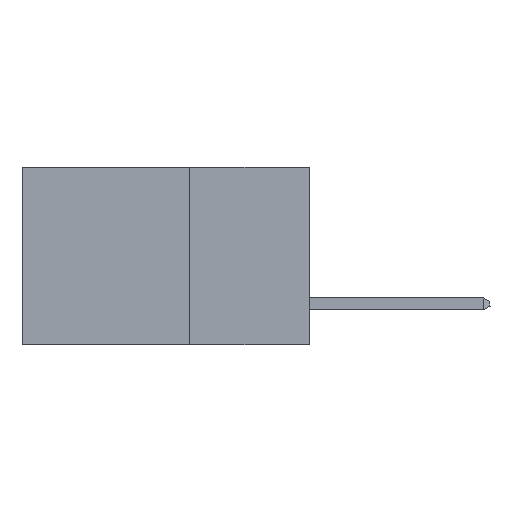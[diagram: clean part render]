
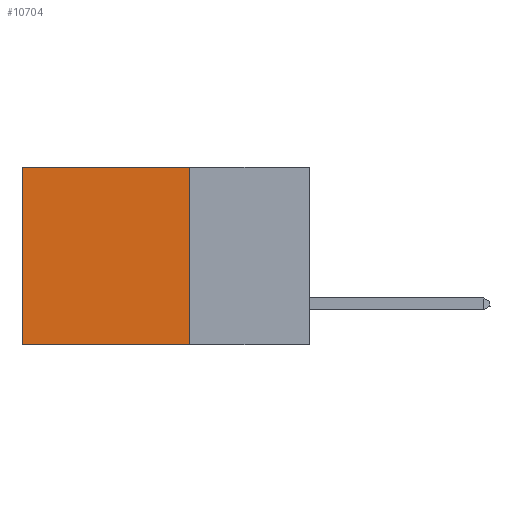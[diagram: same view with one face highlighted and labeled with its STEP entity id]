
A CAD part, left-side view. The second image highlights one B-rep face of the part: STEP entity #10704.
In plain terms, the highlighted planar face has unit normal (-1, 0, 0).
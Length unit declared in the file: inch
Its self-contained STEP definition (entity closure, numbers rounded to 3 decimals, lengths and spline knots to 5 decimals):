
#724 = LINE ( 'NONE', #19006, #25003 ) ;
#841 = CARTESIAN_POINT ( 'NONE',  ( 0.2875, 0.6, 0. ) ) ;
#2384 = CARTESIAN_POINT ( 'NONE',  ( 0.2875, 0.25, 0. ) ) ;
#4241 = ORIENTED_EDGE ( 'NONE', *, *, #12187, .T. ) ;
#4964 = VERTEX_POINT ( 'NONE', #38207 ) ;
#5717 = DIRECTION ( 'NONE',  ( 0., 0., -1. ) ) ;
#5896 = CARTESIAN_POINT ( 'NONE',  ( 0.2875, 0.25, -0.37 ) ) ;
#7204 = DIRECTION ( 'NONE',  ( 0., 1., 0. ) ) ;
#9213 = VERTEX_POINT ( 'NONE', #10234 ) ;
#10234 = CARTESIAN_POINT ( 'NONE',  ( 0.2875, 0.25, -0.37 ) ) ;
#10535 = VECTOR ( 'NONE', #20836, 39.37008 ) ;
#10704 = ADVANCED_FACE ( 'NONE', ( #17303 ), #29301, .F. ) ;
#11171 = CARTESIAN_POINT ( 'NONE',  ( 0.2875, 0.25, 0. ) ) ;
#11302 = VECTOR ( 'NONE', #21482, 39.37008 ) ;
#12187 = EDGE_CURVE ( 'NONE', #28673, #31275, #12631, .T. ) ;
#12631 = LINE ( 'NONE', #841, #11302 ) ;
#12704 = LINE ( 'NONE', #5896, #10535 ) ;
#15066 = VECTOR ( 'NONE', #22585, 39.37008 ) ;
#15431 = ORIENTED_EDGE ( 'NONE', *, *, #24665, .T. ) ;
#17303 = FACE_OUTER_BOUND ( 'NONE', #21551, .T. ) ;
#19006 = CARTESIAN_POINT ( 'NONE',  ( 0.2875, 0.25, 0. ) ) ;
#19145 = CARTESIAN_POINT ( 'NONE',  ( 0.2875, 0.6, 0. ) ) ;
#19817 = LINE ( 'NONE', #11171, #15066 ) ;
#20836 = DIRECTION ( 'NONE',  ( 0., 1., 0. ) ) ;
#21482 = DIRECTION ( 'NONE',  ( 0., 0., -1. ) ) ;
#21551 = EDGE_LOOP ( 'NONE', ( #4241, #22444, #23532, #15431 ) ) ;
#22118 = CARTESIAN_POINT ( 'NONE',  ( 0.2875, 0.6, -0.37 ) ) ;
#22444 = ORIENTED_EDGE ( 'NONE', *, *, #22811, .F. ) ;
#22585 = DIRECTION ( 'NONE',  ( 0., 0., -1. ) ) ;
#22811 = EDGE_CURVE ( 'NONE', #9213, #31275, #12704, .T. ) ;
#23532 = ORIENTED_EDGE ( 'NONE', *, *, #38141, .F. ) ;
#24665 = EDGE_CURVE ( 'NONE', #4964, #28673, #724, .T. ) ;
#25003 = VECTOR ( 'NONE', #7204, 39.37008 ) ;
#28673 = VERTEX_POINT ( 'NONE', #19145 ) ;
#29301 = PLANE ( 'NONE',  #30901 ) ;
#30901 = AXIS2_PLACEMENT_3D ( 'NONE', #2384, #33225, #5717 ) ;
#31275 = VERTEX_POINT ( 'NONE', #22118 ) ;
#33225 = DIRECTION ( 'NONE',  ( 1., 0., 0. ) ) ;
#38141 = EDGE_CURVE ( 'NONE', #4964, #9213, #19817, .T. ) ;
#38207 = CARTESIAN_POINT ( 'NONE',  ( 0.2875, 0.25, 0. ) ) ;
